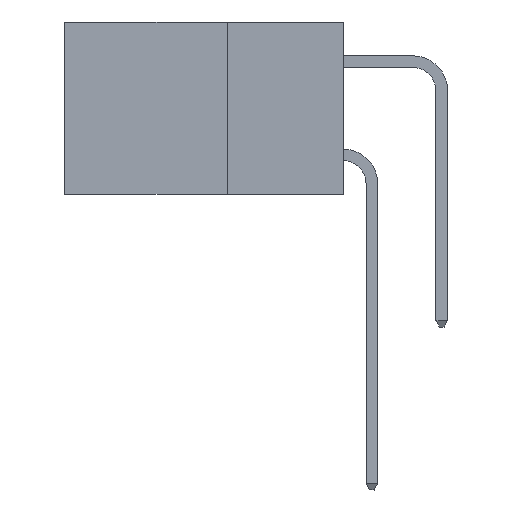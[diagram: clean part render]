
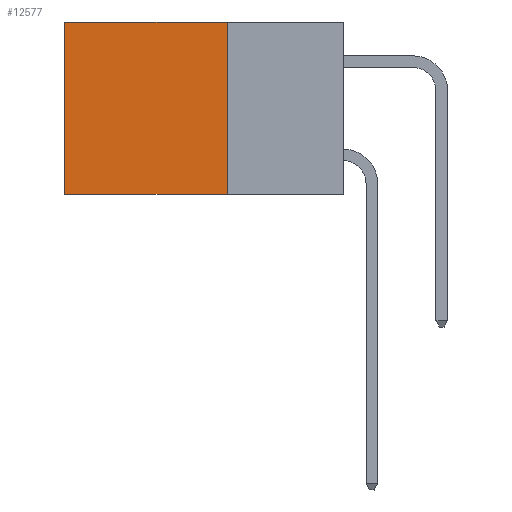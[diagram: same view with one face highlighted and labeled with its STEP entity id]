
A CAD part, left-side view. The second image highlights one B-rep face of the part: STEP entity #12577.
In plain terms, the highlighted planar face has unit normal (-1, 0, 0).
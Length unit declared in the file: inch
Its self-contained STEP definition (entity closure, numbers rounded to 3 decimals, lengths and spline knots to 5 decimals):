
#1069 = CARTESIAN_POINT ( 'NONE',  ( 0.298, 0.25, 0. ) ) ;
#1376 = DIRECTION ( 'NONE',  ( 0., 1., 0. ) ) ;
#1379 = DIRECTION ( 'NONE',  ( 0., 0., -1. ) ) ;
#1909 = CARTESIAN_POINT ( 'NONE',  ( 0.298, 0.25, -0.37 ) ) ;
#2471 = CARTESIAN_POINT ( 'NONE',  ( 0.298, 0.25, 0. ) ) ;
#2616 = CARTESIAN_POINT ( 'NONE',  ( 0.298, 0.6, 0. ) ) ;
#2984 = VECTOR ( 'NONE', #1376, 39.37008 ) ;
#3262 = VECTOR ( 'NONE', #3663, 39.37008 ) ;
#3525 = EDGE_CURVE ( 'NONE', #12849, #7099, #20046, .T. ) ;
#3663 = DIRECTION ( 'NONE',  ( 0., 0., -1. ) ) ;
#4904 = EDGE_CURVE ( 'NONE', #8893, #12849, #15545, .T. ) ;
#5161 = CARTESIAN_POINT ( 'NONE',  ( 0.298, 0.6, 0. ) ) ;
#5467 = DIRECTION ( 'NONE',  ( 0., 0., -1. ) ) ;
#5976 = LINE ( 'NONE', #1909, #17353 ) ;
#6143 = PLANE ( 'NONE',  #6707 ) ;
#6707 = AXIS2_PLACEMENT_3D ( 'NONE', #9332, #10881, #1379 ) ;
#6887 = VERTEX_POINT ( 'NONE', #20163 ) ;
#7099 = VERTEX_POINT ( 'NONE', #13640 ) ;
#8303 = EDGE_CURVE ( 'NONE', #8893, #6887, #11734, .T. ) ;
#8893 = VERTEX_POINT ( 'NONE', #2471 ) ;
#9136 = FACE_OUTER_BOUND ( 'NONE', #15465, .T. ) ;
#9332 = CARTESIAN_POINT ( 'NONE',  ( 0.298, 0.25, 0. ) ) ;
#9949 = DIRECTION ( 'NONE',  ( 0., 1., 0. ) ) ;
#10791 = EDGE_CURVE ( 'NONE', #6887, #7099, #5976, .T. ) ;
#10881 = DIRECTION ( 'NONE',  ( 1., 0., 0. ) ) ;
#11520 = VECTOR ( 'NONE', #5467, 39.37008 ) ;
#11734 = LINE ( 'NONE', #16129, #3262 ) ;
#12577 = ADVANCED_FACE ( 'NONE', ( #9136 ), #6143, .F. ) ;
#12849 = VERTEX_POINT ( 'NONE', #5161 ) ;
#13640 = CARTESIAN_POINT ( 'NONE',  ( 0.298, 0.6, -0.37 ) ) ;
#14667 = ORIENTED_EDGE ( 'NONE', *, *, #10791, .F. ) ;
#15465 = EDGE_LOOP ( 'NONE', ( #19537, #14667, #19303, #18166 ) ) ;
#15545 = LINE ( 'NONE', #1069, #2984 ) ;
#16129 = CARTESIAN_POINT ( 'NONE',  ( 0.298, 0.25, 0. ) ) ;
#17353 = VECTOR ( 'NONE', #9949, 39.37008 ) ;
#18166 = ORIENTED_EDGE ( 'NONE', *, *, #4904, .T. ) ;
#19303 = ORIENTED_EDGE ( 'NONE', *, *, #8303, .F. ) ;
#19537 = ORIENTED_EDGE ( 'NONE', *, *, #3525, .T. ) ;
#20046 = LINE ( 'NONE', #2616, #11520 ) ;
#20163 = CARTESIAN_POINT ( 'NONE',  ( 0.298, 0.25, -0.37 ) ) ;
